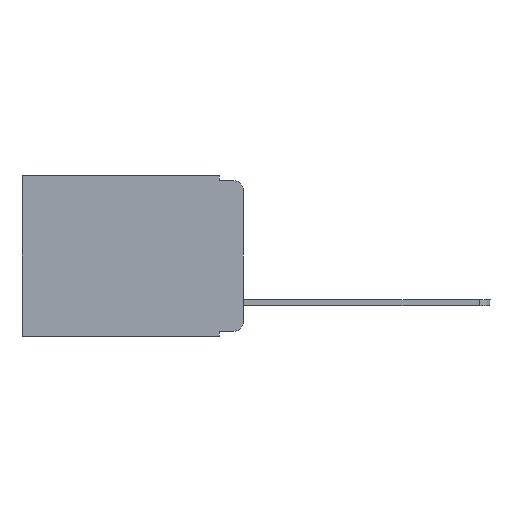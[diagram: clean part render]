
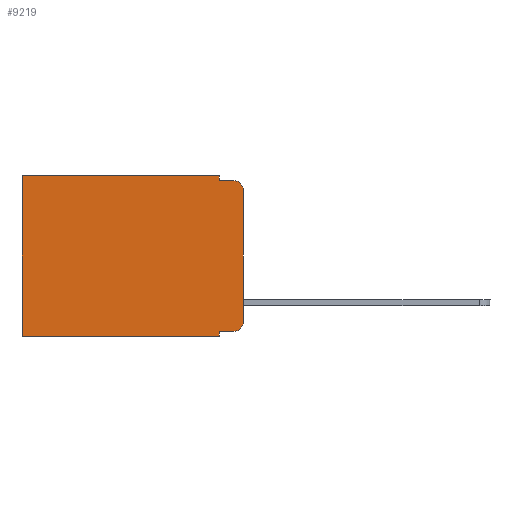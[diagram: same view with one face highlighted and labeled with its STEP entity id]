
A CAD part, left-side view. The second image highlights one B-rep face of the part: STEP entity #9219.
In plain terms, the highlighted planar face has unit normal (-1, 0, 0).
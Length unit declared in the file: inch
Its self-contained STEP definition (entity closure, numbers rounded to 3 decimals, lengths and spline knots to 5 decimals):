
#123 = ORIENTED_EDGE ( 'NONE', *, *, #127, .F. ) ;
#127 = EDGE_CURVE ( 'NONE', #3942, #6121, #1437, .T. ) ;
#147 = CARTESIAN_POINT ( 'NONE',  ( 0.298, 0.02, -0.03 ) ) ;
#494 = CARTESIAN_POINT ( 'NONE',  ( 0.298, 0.051, 0. ) ) ;
#508 = ORIENTED_EDGE ( 'NONE', *, *, #6123, .F. ) ;
#536 = CARTESIAN_POINT ( 'NONE',  ( 0.298, 0.051, -0.333 ) ) ;
#681 = DIRECTION ( 'NONE',  ( 0., 0., -1. ) ) ;
#746 = CARTESIAN_POINT ( 'NONE',  ( 0.298, 0.051, -0.01 ) ) ;
#864 = DIRECTION ( 'NONE',  ( 0., 0., -1. ) ) ;
#921 = CARTESIAN_POINT ( 'NONE',  ( 0.298, 0.02, -0.333 ) ) ;
#935 = VERTEX_POINT ( 'NONE', #4131 ) ;
#1093 = CARTESIAN_POINT ( 'NONE',  ( 0.298, 0.02, -0.313 ) ) ;
#1219 = EDGE_CURVE ( 'NONE', #8968, #2364, #2514, .T. ) ;
#1232 = LINE ( 'NONE', #3236, #4681 ) ;
#1379 = CARTESIAN_POINT ( 'NONE',  ( 0.298, 0.051, -0.333 ) ) ;
#1437 = LINE ( 'NONE', #7200, #4921 ) ;
#1596 = LINE ( 'NONE', #2198, #3139 ) ;
#1605 = DIRECTION ( 'NONE',  ( -1., 0., 0. ) ) ;
#1764 = VERTEX_POINT ( 'NONE', #3485 ) ;
#1801 = LINE ( 'NONE', #536, #3024 ) ;
#2198 = CARTESIAN_POINT ( 'NONE',  ( 0.298, 0.051, -0.01 ) ) ;
#2311 = LINE ( 'NONE', #4473, #6423 ) ;
#2364 = VERTEX_POINT ( 'NONE', #4230 ) ;
#2514 = LINE ( 'NONE', #6134, #6981 ) ;
#2535 = DIRECTION ( 'NONE',  ( -1., 0., 0. ) ) ;
#2635 = DIRECTION ( 'NONE',  ( 0., 0., -1. ) ) ;
#2697 = AXIS2_PLACEMENT_3D ( 'NONE', #147, #1605, #681 ) ;
#2870 = VERTEX_POINT ( 'NONE', #5300 ) ;
#2906 = DIRECTION ( 'NONE',  ( 0., 1., 0. ) ) ;
#2976 = DIRECTION ( 'NONE',  ( 0., 0., -1. ) ) ;
#3024 = VECTOR ( 'NONE', #7526, 39.37008 ) ;
#3100 = DIRECTION ( 'NONE',  ( 0., 0., -1. ) ) ;
#3139 = VECTOR ( 'NONE', #7266, 39.37008 ) ;
#3236 = CARTESIAN_POINT ( 'NONE',  ( 0.298, 0.473, 0. ) ) ;
#3342 = ORIENTED_EDGE ( 'NONE', *, *, #7710, .T. ) ;
#3485 = CARTESIAN_POINT ( 'NONE',  ( 0.298, 0.473, 0. ) ) ;
#3720 = EDGE_LOOP ( 'NONE', ( #5811, #4716, #508, #123, #8695, #4868, #6710, #6833, #4108, #3342 ) ) ;
#3725 = PLANE ( 'NONE',  #6012 ) ;
#3917 = CIRCLE ( 'NONE', #8727, 0.02 ) ;
#3942 = VERTEX_POINT ( 'NONE', #6540 ) ;
#3971 = EDGE_CURVE ( 'NONE', #2870, #935, #2311, .T. ) ;
#4108 = ORIENTED_EDGE ( 'NONE', *, *, #8131, .T. ) ;
#4120 = DIRECTION ( 'NONE',  ( 0., 0., -1. ) ) ;
#4131 = CARTESIAN_POINT ( 'NONE',  ( 0.298, 0., -0.313 ) ) ;
#4230 = CARTESIAN_POINT ( 'NONE',  ( 0.298, 0.473, -0.343 ) ) ;
#4473 = CARTESIAN_POINT ( 'NONE',  ( 0.298, 0., 0. ) ) ;
#4681 = VECTOR ( 'NONE', #6156, 39.37008 ) ;
#4716 = ORIENTED_EDGE ( 'NONE', *, *, #5744, .T. ) ;
#4752 = VERTEX_POINT ( 'NONE', #7883 ) ;
#4868 = ORIENTED_EDGE ( 'NONE', *, *, #8460, .T. ) ;
#4921 = VECTOR ( 'NONE', #864, 39.37008 ) ;
#5151 = DIRECTION ( 'NONE',  ( 1., 0., 0. ) ) ;
#5300 = CARTESIAN_POINT ( 'NONE',  ( 0.298, 0., -0.03 ) ) ;
#5744 = EDGE_CURVE ( 'NONE', #2870, #4752, #7512, .T. ) ;
#5803 = FACE_OUTER_BOUND ( 'NONE', #3720, .T. ) ;
#5811 = ORIENTED_EDGE ( 'NONE', *, *, #3971, .F. ) ;
#5813 = CARTESIAN_POINT ( 'NONE',  ( 0.298, 0., 0. ) ) ;
#6012 = AXIS2_PLACEMENT_3D ( 'NONE', #6555, #5151, #2976 ) ;
#6027 = VECTOR ( 'NONE', #2635, 39.37008 ) ;
#6121 = VERTEX_POINT ( 'NONE', #746 ) ;
#6123 = EDGE_CURVE ( 'NONE', #6121, #4752, #1596, .T. ) ;
#6134 = CARTESIAN_POINT ( 'NONE',  ( 0.298, 0., -0.343 ) ) ;
#6156 = DIRECTION ( 'NONE',  ( 0., 0., -1. ) ) ;
#6423 = VECTOR ( 'NONE', #3100, 39.37008 ) ;
#6540 = CARTESIAN_POINT ( 'NONE',  ( 0.298, 0.051, 0. ) ) ;
#6555 = CARTESIAN_POINT ( 'NONE',  ( 0.298, 0., 0. ) ) ;
#6636 = VERTEX_POINT ( 'NONE', #921 ) ;
#6640 = VECTOR ( 'NONE', #2906, 39.37008 ) ;
#6710 = ORIENTED_EDGE ( 'NONE', *, *, #1219, .F. ) ;
#6833 = ORIENTED_EDGE ( 'NONE', *, *, #8088, .F. ) ;
#6917 = LINE ( 'NONE', #494, #6027 ) ;
#6981 = VECTOR ( 'NONE', #9007, 39.37008 ) ;
#7200 = CARTESIAN_POINT ( 'NONE',  ( 0.298, 0.051, 0. ) ) ;
#7266 = DIRECTION ( 'NONE',  ( 0., -1., 0. ) ) ;
#7360 = LINE ( 'NONE', #5813, #6640 ) ;
#7440 = VERTEX_POINT ( 'NONE', #1379 ) ;
#7512 = CIRCLE ( 'NONE', #2697, 0.02 ) ;
#7526 = DIRECTION ( 'NONE',  ( 0., -1., 0. ) ) ;
#7552 = CARTESIAN_POINT ( 'NONE',  ( 0.298, 0.051, -0.343 ) ) ;
#7710 = EDGE_CURVE ( 'NONE', #6636, #935, #3917, .T. ) ;
#7883 = CARTESIAN_POINT ( 'NONE',  ( 0.298, 0.02, -0.01 ) ) ;
#8088 = EDGE_CURVE ( 'NONE', #7440, #8968, #6917, .T. ) ;
#8131 = EDGE_CURVE ( 'NONE', #7440, #6636, #1801, .T. ) ;
#8460 = EDGE_CURVE ( 'NONE', #1764, #2364, #1232, .T. ) ;
#8695 = ORIENTED_EDGE ( 'NONE', *, *, #8759, .T. ) ;
#8727 = AXIS2_PLACEMENT_3D ( 'NONE', #1093, #2535, #4120 ) ;
#8759 = EDGE_CURVE ( 'NONE', #3942, #1764, #7360, .T. ) ;
#8968 = VERTEX_POINT ( 'NONE', #7552 ) ;
#9007 = DIRECTION ( 'NONE',  ( 0., 1., 0. ) ) ;
#9219 = ADVANCED_FACE ( 'NONE', ( #5803 ), #3725, .F. ) ;
